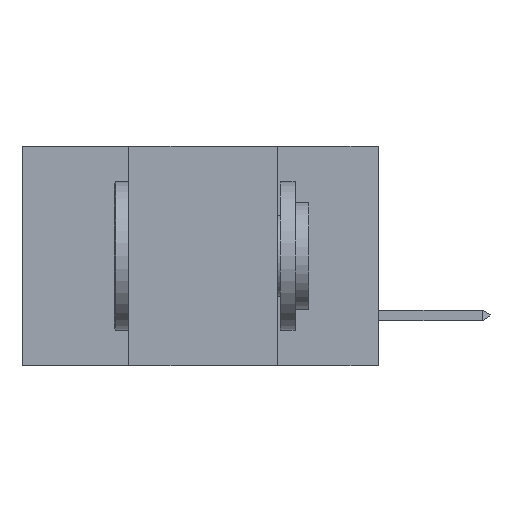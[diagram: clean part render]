
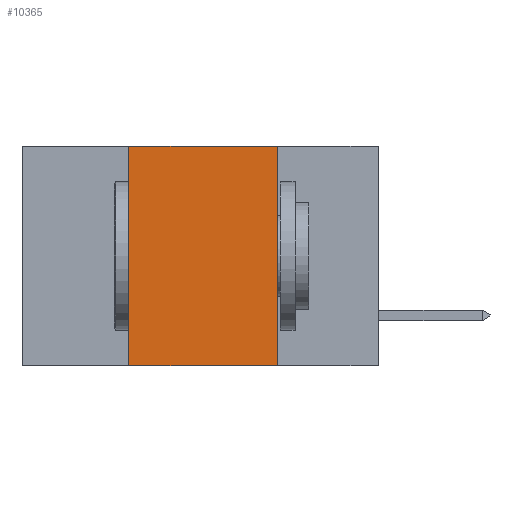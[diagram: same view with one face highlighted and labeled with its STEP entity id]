
A CAD part, left-side view. The second image highlights one B-rep face of the part: STEP entity #10365.
In plain terms, the highlighted planar face has unit normal (-1, 0, 0).
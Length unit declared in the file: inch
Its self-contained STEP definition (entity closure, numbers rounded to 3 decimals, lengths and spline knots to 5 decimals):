
#590 = CARTESIAN_POINT ( 'NONE',  ( 0., 0.6, -0.37 ) ) ;
#973 = VECTOR ( 'NONE', #11489, 39.37008 ) ;
#1629 = CARTESIAN_POINT ( 'NONE',  ( 0., 0.17, 0. ) ) ;
#1695 = AXIS2_PLACEMENT_3D ( 'NONE', #5314, #6630, #4048 ) ;
#1895 = DIRECTION ( 'NONE',  ( 0., 0., 1. ) ) ;
#2735 = ORIENTED_EDGE ( 'NONE', *, *, #7928, .T. ) ;
#2798 = FACE_OUTER_BOUND ( 'NONE', #11895, .T. ) ;
#3866 = VECTOR ( 'NONE', #13459, 39.37008 ) ;
#4048 = DIRECTION ( 'NONE',  ( 0., 0., -1. ) ) ;
#5314 = CARTESIAN_POINT ( 'NONE',  ( 0., 0.6, 0. ) ) ;
#5465 = CARTESIAN_POINT ( 'NONE',  ( 0., 0.42, 0. ) ) ;
#6070 = VECTOR ( 'NONE', #10451, 39.37008 ) ;
#6239 = EDGE_CURVE ( 'NONE', #6460, #9266, #13059, .T. ) ;
#6460 = VERTEX_POINT ( 'NONE', #7955 ) ;
#6630 = DIRECTION ( 'NONE',  ( 1., 0., 0. ) ) ;
#6991 = CARTESIAN_POINT ( 'NONE',  ( 0., 0.6, 0. ) ) ;
#7608 = CARTESIAN_POINT ( 'NONE',  ( 0., 0.42, -0.37 ) ) ;
#7928 = EDGE_CURVE ( 'NONE', #14975, #9266, #9074, .T. ) ;
#7955 = CARTESIAN_POINT ( 'NONE',  ( 0., 0.17, 0. ) ) ;
#8126 = EDGE_CURVE ( 'NONE', #14975, #12721, #10987, .T. ) ;
#8435 = EDGE_CURVE ( 'NONE', #12721, #6460, #15032, .T. ) ;
#8441 = ORIENTED_EDGE ( 'NONE', *, *, #8435, .F. ) ;
#9074 = LINE ( 'NONE', #590, #973 ) ;
#9266 = VERTEX_POINT ( 'NONE', #15497 ) ;
#9472 = VECTOR ( 'NONE', #1895, 39.37008 ) ;
#9660 = PLANE ( 'NONE',  #1695 ) ;
#10365 = ADVANCED_FACE ( 'NONE', ( #2798 ), #9660, .F. ) ;
#10451 = DIRECTION ( 'NONE',  ( 0., -1., 0. ) ) ;
#10987 = LINE ( 'NONE', #5465, #9472 ) ;
#11288 = ORIENTED_EDGE ( 'NONE', *, *, #6239, .F. ) ;
#11489 = DIRECTION ( 'NONE',  ( 0., -1., 0. ) ) ;
#11895 = EDGE_LOOP ( 'NONE', ( #11288, #8441, #15304, #2735 ) ) ;
#12721 = VERTEX_POINT ( 'NONE', #13331 ) ;
#13059 = LINE ( 'NONE', #1629, #3866 ) ;
#13331 = CARTESIAN_POINT ( 'NONE',  ( 0., 0.42, 0. ) ) ;
#13459 = DIRECTION ( 'NONE',  ( 0., 0., -1. ) ) ;
#14975 = VERTEX_POINT ( 'NONE', #7608 ) ;
#15032 = LINE ( 'NONE', #6991, #6070 ) ;
#15304 = ORIENTED_EDGE ( 'NONE', *, *, #8126, .F. ) ;
#15497 = CARTESIAN_POINT ( 'NONE',  ( 0., 0.17, -0.37 ) ) ;
